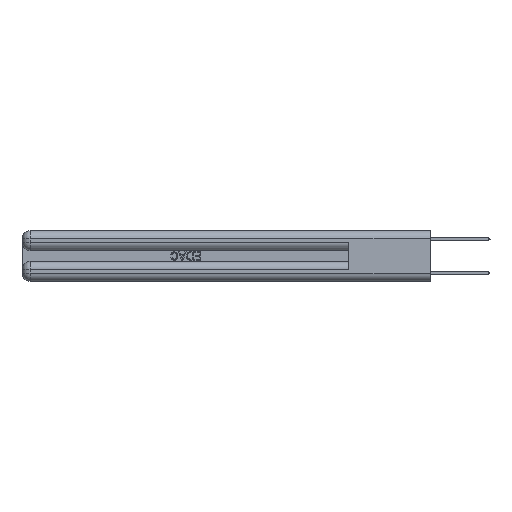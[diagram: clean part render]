
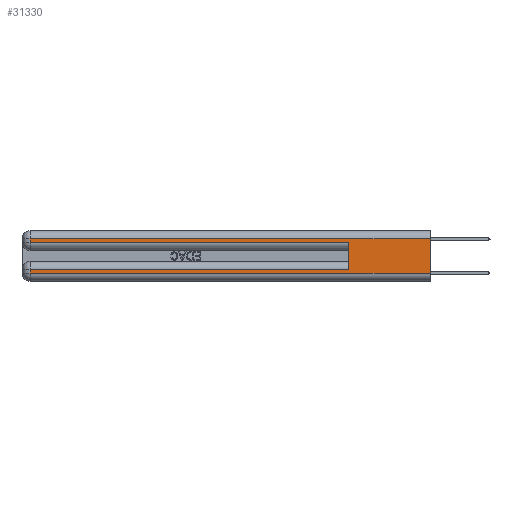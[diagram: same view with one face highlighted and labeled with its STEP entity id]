
A CAD part, left-side view. The second image highlights one B-rep face of the part: STEP entity #31330.
In plain terms, the highlighted planar face has unit normal (-1, 0, 0).
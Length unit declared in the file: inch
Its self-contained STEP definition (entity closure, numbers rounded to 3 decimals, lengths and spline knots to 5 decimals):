
#646 = VERTEX_POINT ( 'NONE', #30003 ) ;
#968 = DIRECTION ( 'NONE',  ( 1., 0., 0. ) ) ;
#1141 = CARTESIAN_POINT ( 'NONE',  ( 0., 0.6, 0.285 ) ) ;
#1557 = VERTEX_POINT ( 'NONE', #12363 ) ;
#1807 = LINE ( 'NONE', #5365, #11012 ) ;
#2694 = CARTESIAN_POINT ( 'NONE',  ( 0., 0.6, 0.085 ) ) ;
#2898 = LINE ( 'NONE', #11985, #29270 ) ;
#3039 = CARTESIAN_POINT ( 'NONE',  ( 0., 2.94, 0.31 ) ) ;
#3048 = ORIENTED_EDGE ( 'NONE', *, *, #23081, .F. ) ;
#3680 = ORIENTED_EDGE ( 'NONE', *, *, #11103, .T. ) ;
#3769 = CARTESIAN_POINT ( 'NONE',  ( 0., 0., 0.37 ) ) ;
#4807 = VERTEX_POINT ( 'NONE', #29559 ) ;
#5249 = EDGE_CURVE ( 'NONE', #646, #14738, #21258, .T. ) ;
#5365 = CARTESIAN_POINT ( 'NONE',  ( 0., 0., 0.31 ) ) ;
#7427 = CARTESIAN_POINT ( 'NONE',  ( 0., 0., 0.06 ) ) ;
#7561 = VERTEX_POINT ( 'NONE', #29586 ) ;
#7946 = LINE ( 'NONE', #24928, #12155 ) ;
#8592 = PLANE ( 'NONE',  #19085 ) ;
#9434 = DIRECTION ( 'NONE',  ( 0., 0., -1. ) ) ;
#9791 = EDGE_CURVE ( 'NONE', #4807, #14738, #26368, .T. ) ;
#10191 = DIRECTION ( 'NONE',  ( 0., 1., 0. ) ) ;
#11003 = DIRECTION ( 'NONE',  ( 0., 0., 1. ) ) ;
#11012 = VECTOR ( 'NONE', #15204, 39.37008 ) ;
#11103 = EDGE_CURVE ( 'NONE', #14966, #1557, #7946, .T. ) ;
#11157 = EDGE_CURVE ( 'NONE', #4807, #23487, #1807, .T. ) ;
#11546 = CARTESIAN_POINT ( 'NONE',  ( 0., 0., 0.37 ) ) ;
#11985 = CARTESIAN_POINT ( 'NONE',  ( 0., 0., 0.285 ) ) ;
#12155 = VECTOR ( 'NONE', #10191, 39.37008 ) ;
#12363 = CARTESIAN_POINT ( 'NONE',  ( 0., 2.94, 0.085 ) ) ;
#13553 = FACE_OUTER_BOUND ( 'NONE', #24223, .T. ) ;
#14017 = VECTOR ( 'NONE', #31313, 39.37008 ) ;
#14732 = ORIENTED_EDGE ( 'NONE', *, *, #9791, .F. ) ;
#14738 = VERTEX_POINT ( 'NONE', #7427 ) ;
#14966 = VERTEX_POINT ( 'NONE', #2694 ) ;
#15204 = DIRECTION ( 'NONE',  ( 0., 1., 0. ) ) ;
#15300 = EDGE_CURVE ( 'NONE', #1557, #646, #18754, .T. ) ;
#15331 = VECTOR ( 'NONE', #9434, 39.37008 ) ;
#15671 = ORIENTED_EDGE ( 'NONE', *, *, #15300, .T. ) ;
#16520 = CARTESIAN_POINT ( 'NONE',  ( 0., 0., 0.06 ) ) ;
#18253 = EDGE_CURVE ( 'NONE', #7561, #24969, #2898, .T. ) ;
#18322 = VECTOR ( 'NONE', #31143, 39.37008 ) ;
#18358 = CARTESIAN_POINT ( 'NONE',  ( 0., 0.6, 0.145 ) ) ;
#18704 = LINE ( 'NONE', #18358, #29405 ) ;
#18754 = LINE ( 'NONE', #24057, #15331 ) ;
#19085 = AXIS2_PLACEMENT_3D ( 'NONE', #3769, #968, #25581 ) ;
#21258 = LINE ( 'NONE', #16520, #14017 ) ;
#23081 = EDGE_CURVE ( 'NONE', #14966, #24969, #18704, .T. ) ;
#23475 = DIRECTION ( 'NONE',  ( 0., 0., -1. ) ) ;
#23487 = VERTEX_POINT ( 'NONE', #3039 ) ;
#23802 = ORIENTED_EDGE ( 'NONE', *, *, #28690, .T. ) ;
#24057 = CARTESIAN_POINT ( 'NONE',  ( 0., 2.94, 0.37 ) ) ;
#24223 = EDGE_LOOP ( 'NONE', ( #14732, #24658, #23802, #24904, #3048, #3680, #15671, #27411 ) ) ;
#24658 = ORIENTED_EDGE ( 'NONE', *, *, #11157, .T. ) ;
#24904 = ORIENTED_EDGE ( 'NONE', *, *, #18253, .T. ) ;
#24928 = CARTESIAN_POINT ( 'NONE',  ( 0., 0., 0.085 ) ) ;
#24969 = VERTEX_POINT ( 'NONE', #1141 ) ;
#25581 = DIRECTION ( 'NONE',  ( 0., 0., -1. ) ) ;
#26368 = LINE ( 'NONE', #11546, #18322 ) ;
#26373 = VECTOR ( 'NONE', #23475, 39.37008 ) ;
#27245 = DIRECTION ( 'NONE',  ( 0., -1., 0. ) ) ;
#27411 = ORIENTED_EDGE ( 'NONE', *, *, #5249, .T. ) ;
#28690 = EDGE_CURVE ( 'NONE', #23487, #7561, #29028, .T. ) ;
#29028 = LINE ( 'NONE', #30997, #26373 ) ;
#29270 = VECTOR ( 'NONE', #27245, 39.37008 ) ;
#29405 = VECTOR ( 'NONE', #11003, 39.37008 ) ;
#29559 = CARTESIAN_POINT ( 'NONE',  ( 0., 0., 0.31 ) ) ;
#29586 = CARTESIAN_POINT ( 'NONE',  ( 0., 2.94, 0.285 ) ) ;
#30003 = CARTESIAN_POINT ( 'NONE',  ( 0., 2.94, 0.06 ) ) ;
#30997 = CARTESIAN_POINT ( 'NONE',  ( 0., 2.94, 0.37 ) ) ;
#31143 = DIRECTION ( 'NONE',  ( 0., 0., -1. ) ) ;
#31313 = DIRECTION ( 'NONE',  ( 0., -1., 0. ) ) ;
#31330 = ADVANCED_FACE ( 'NONE', ( #13553 ), #8592, .F. ) ;
